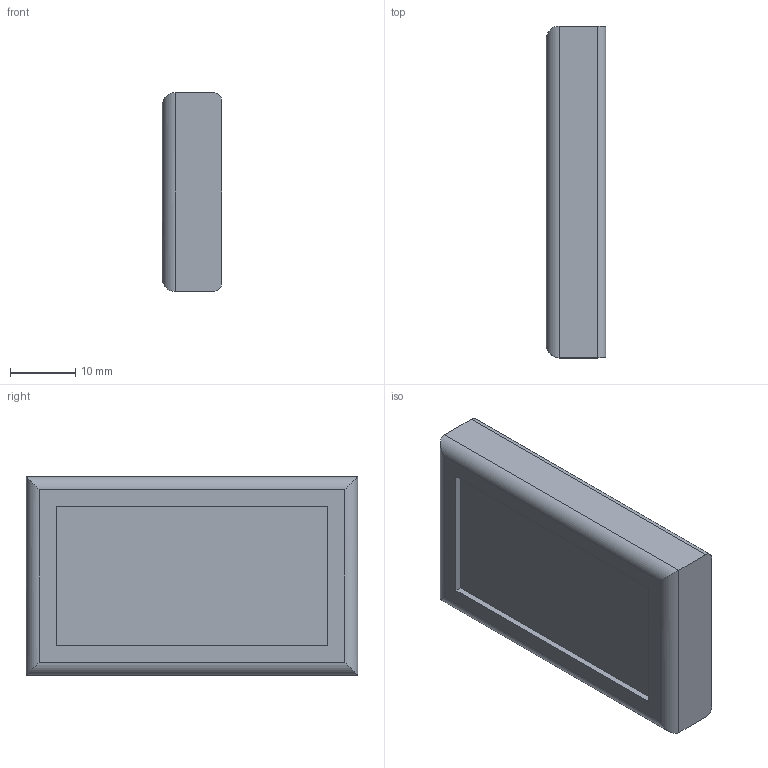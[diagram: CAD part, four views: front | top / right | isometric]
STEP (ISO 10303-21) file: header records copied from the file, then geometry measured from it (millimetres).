
FILE_DESCRIPTION (( 'STEP AP214' ), '1' );
FILE_NAME ('magplate.STEP', '2013-11-06T01:46:48', ( '' ), ( '' ), 'SwSTEP 2.0', 'SolidWorks 2013', '' );
FILE_SCHEMA (( 'AUTOMOTIVE_DESIGN' ));
Length unit declared in the file: inch
Products named in the file (1): magplate
Bounding box: 9.14 x 50.8 x 30.48 mm (x, y, z)
Volume: 8409.1 mm3; surface area: 5147.8 mm2
Topology: 1 solids, 1 shells, 25 faces, 62 edges, 40 vertices
Faces by surface type: plane 19, cylinder 6
Entity records: 768 total; most frequent: CARTESIAN_POINT 140, ORIENTED_EDGE 124, DIRECTION 114, EDGE_CURVE 62, LINE 54, VECTOR 54, VERTEX_POINT 40, AXIS2_PLACEMENT_3D 30
